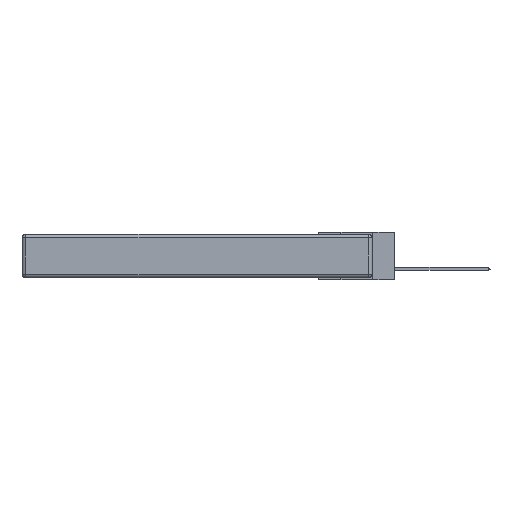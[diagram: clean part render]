
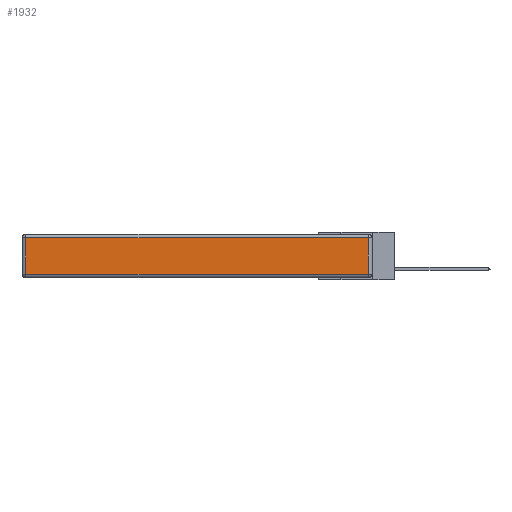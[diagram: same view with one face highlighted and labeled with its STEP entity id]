
A CAD part, left-side view. The second image highlights one B-rep face of the part: STEP entity #1932.
In plain terms, the highlighted planar face has unit normal (-1, 0, 0).
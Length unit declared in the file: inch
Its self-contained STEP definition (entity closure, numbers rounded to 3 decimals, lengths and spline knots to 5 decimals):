
#1743 = DIRECTION ( 'NONE',  ( 0., -1., 0. ) ) ;
#1932 = ADVANCED_FACE ( 'NONE', ( #27071 ), #19294, .T. ) ;
#2126 = CARTESIAN_POINT ( 'NONE',  ( 0., 0.03, -0.313 ) ) ;
#3202 = EDGE_CURVE ( 'NONE', #26076, #22006, #20038, .T. ) ;
#3628 = CARTESIAN_POINT ( 'NONE',  ( 0., 2.75, -0.03 ) ) ;
#3999 = ORIENTED_EDGE ( 'NONE', *, *, #7403, .T. ) ;
#5144 = DIRECTION ( 'NONE',  ( 0., 0., 1. ) ) ;
#5547 = VECTOR ( 'NONE', #5144, 39.37008 ) ;
#5567 = CARTESIAN_POINT ( 'NONE',  ( 0., 0.03, -0.343 ) ) ;
#6690 = EDGE_LOOP ( 'NONE', ( #8039, #3999, #6905, #21092 ) ) ;
#6905 = ORIENTED_EDGE ( 'NONE', *, *, #30708, .T. ) ;
#7403 = EDGE_CURVE ( 'NONE', #22006, #10508, #14129, .T. ) ;
#8039 = ORIENTED_EDGE ( 'NONE', *, *, #3202, .T. ) ;
#10508 = VERTEX_POINT ( 'NONE', #14256 ) ;
#14129 = LINE ( 'NONE', #5567, #5547 ) ;
#14256 = CARTESIAN_POINT ( 'NONE',  ( 0., 0.03, -0.03 ) ) ;
#15013 = CARTESIAN_POINT ( 'NONE',  ( 0., 2.72, -0.313 ) ) ;
#15626 = VECTOR ( 'NONE', #30337, 39.37008 ) ;
#15985 = DIRECTION ( 'NONE',  ( 0., 0., -1. ) ) ;
#16043 = EDGE_CURVE ( 'NONE', #29018, #26076, #30905, .T. ) ;
#16306 = AXIS2_PLACEMENT_3D ( 'NONE', #21614, #18981, #19180 ) ;
#18513 = VECTOR ( 'NONE', #15985, 39.37008 ) ;
#18981 = DIRECTION ( 'NONE',  ( -1., 0., 0. ) ) ;
#19180 = DIRECTION ( 'NONE',  ( 0., 0., 1. ) ) ;
#19294 = PLANE ( 'NONE',  #16306 ) ;
#20038 = LINE ( 'NONE', #30667, #23414 ) ;
#21092 = ORIENTED_EDGE ( 'NONE', *, *, #16043, .T. ) ;
#21482 = CARTESIAN_POINT ( 'NONE',  ( 0., 2.72, -0.03 ) ) ;
#21614 = CARTESIAN_POINT ( 'NONE',  ( 0., 0., -0.343 ) ) ;
#22006 = VERTEX_POINT ( 'NONE', #2126 ) ;
#23414 = VECTOR ( 'NONE', #1743, 39.37008 ) ;
#26076 = VERTEX_POINT ( 'NONE', #15013 ) ;
#27071 = FACE_OUTER_BOUND ( 'NONE', #6690, .T. ) ;
#27206 = LINE ( 'NONE', #3628, #15626 ) ;
#27612 = CARTESIAN_POINT ( 'NONE',  ( 0., 2.72, -0.343 ) ) ;
#29018 = VERTEX_POINT ( 'NONE', #21482 ) ;
#30337 = DIRECTION ( 'NONE',  ( 0., 1., 0. ) ) ;
#30667 = CARTESIAN_POINT ( 'NONE',  ( 0., 0., -0.313 ) ) ;
#30708 = EDGE_CURVE ( 'NONE', #10508, #29018, #27206, .T. ) ;
#30905 = LINE ( 'NONE', #27612, #18513 ) ;
